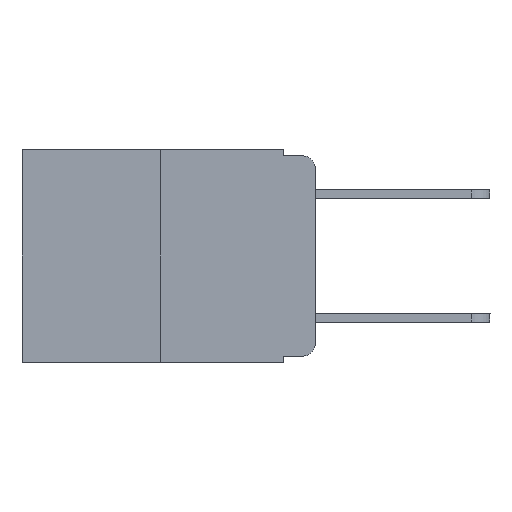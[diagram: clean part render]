
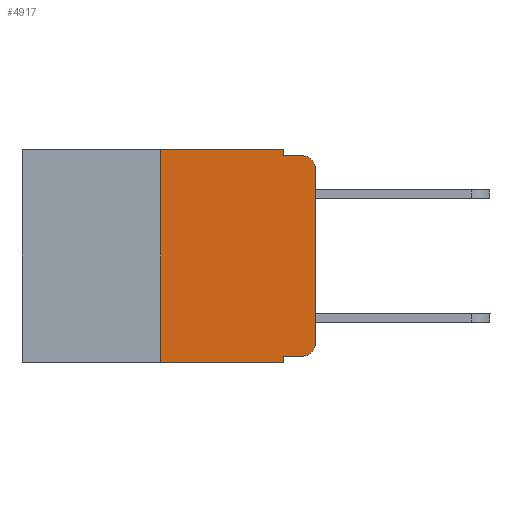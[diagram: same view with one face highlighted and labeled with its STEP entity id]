
A CAD part, left-side view. The second image highlights one B-rep face of the part: STEP entity #4917.
In plain terms, the highlighted planar face has unit normal (-1, 0, 0).
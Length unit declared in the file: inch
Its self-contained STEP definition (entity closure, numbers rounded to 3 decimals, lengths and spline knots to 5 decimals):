
#163 = ORIENTED_EDGE ( 'NONE', *, *, #10493, .F. ) ;
#191 = VERTEX_POINT ( 'NONE', #12729 ) ;
#669 = DIRECTION ( 'NONE',  ( 0., -1., 0. ) ) ;
#799 = VECTOR ( 'NONE', #8525, 39.37008 ) ;
#1104 = CARTESIAN_POINT ( 'NONE',  ( 0., 0.473, 0. ) ) ;
#1194 = ORIENTED_EDGE ( 'NONE', *, *, #16349, .T. ) ;
#1467 = VERTEX_POINT ( 'NONE', #7719 ) ;
#1587 = CARTESIAN_POINT ( 'NONE',  ( 0., 0., -0.03 ) ) ;
#1673 = LINE ( 'NONE', #8542, #1927 ) ;
#1927 = VECTOR ( 'NONE', #15159, 39.37008 ) ;
#2111 = EDGE_LOOP ( 'NONE', ( #20418, #5104, #2732, #8688, #163, #16193, #19515, #16951, #8560, #1194 ) ) ;
#2707 = EDGE_CURVE ( 'NONE', #16683, #191, #2872, .T. ) ;
#2732 = ORIENTED_EDGE ( 'NONE', *, *, #19059, .F. ) ;
#2756 = DIRECTION ( 'NONE',  ( 0., -1., 0. ) ) ;
#2762 = DIRECTION ( 'NONE',  ( 1., 0., 0. ) ) ;
#2872 = LINE ( 'NONE', #6411, #19790 ) ;
#3437 = CARTESIAN_POINT ( 'NONE',  ( 0., 0.051, -0.343 ) ) ;
#4051 = CARTESIAN_POINT ( 'NONE',  ( 0., 0., 0. ) ) ;
#4280 = VERTEX_POINT ( 'NONE', #19044 ) ;
#4456 = PLANE ( 'NONE',  #14859 ) ;
#4917 = ADVANCED_FACE ( 'NONE', ( #21011 ), #4456, .F. ) ;
#5104 = ORIENTED_EDGE ( 'NONE', *, *, #11301, .T. ) ;
#5699 = LINE ( 'NONE', #10876, #12565 ) ;
#5936 = VERTEX_POINT ( 'NONE', #19601 ) ;
#6309 = CARTESIAN_POINT ( 'NONE',  ( 0., 0.051, 0. ) ) ;
#6411 = CARTESIAN_POINT ( 'NONE',  ( 0., 0.25, 0. ) ) ;
#6610 = LINE ( 'NONE', #9608, #7412 ) ;
#6990 = LINE ( 'NONE', #10403, #10577 ) ;
#7412 = VECTOR ( 'NONE', #14306, 39.37008 ) ;
#7543 = LINE ( 'NONE', #12503, #9067 ) ;
#7676 = DIRECTION ( 'NONE',  ( 0., -1., 0. ) ) ;
#7719 = CARTESIAN_POINT ( 'NONE',  ( 0., 0.051, -0.01 ) ) ;
#8001 = CARTESIAN_POINT ( 'NONE',  ( 0., 0.25, -0.343 ) ) ;
#8077 = VERTEX_POINT ( 'NONE', #1587 ) ;
#8152 = DIRECTION ( 'NONE',  ( 0., 0., -1. ) ) ;
#8256 = EDGE_CURVE ( 'NONE', #4280, #21171, #1673, .T. ) ;
#8525 = DIRECTION ( 'NONE',  ( 0., -1., 0. ) ) ;
#8542 = CARTESIAN_POINT ( 'NONE',  ( 0., 0.051, 0. ) ) ;
#8560 = ORIENTED_EDGE ( 'NONE', *, *, #18444, .T. ) ;
#8688 = ORIENTED_EDGE ( 'NONE', *, *, #17361, .F. ) ;
#9067 = VECTOR ( 'NONE', #2756, 39.37008 ) ;
#9608 = CARTESIAN_POINT ( 'NONE',  ( 0., 0.051, 0. ) ) ;
#9983 = VERTEX_POINT ( 'NONE', #6309 ) ;
#10403 = CARTESIAN_POINT ( 'NONE',  ( 0., 0.473, -0.343 ) ) ;
#10416 = CARTESIAN_POINT ( 'NONE',  ( 0., 0.02, -0.01 ) ) ;
#10421 = CARTESIAN_POINT ( 'NONE',  ( 0., 0.473, 0. ) ) ;
#10491 = CARTESIAN_POINT ( 'NONE',  ( 0., 0., -0.313 ) ) ;
#10493 = EDGE_CURVE ( 'NONE', #191, #9983, #14091, .T. ) ;
#10577 = VECTOR ( 'NONE', #669, 39.37008 ) ;
#10876 = CARTESIAN_POINT ( 'NONE',  ( 0., 0.051, -0.01 ) ) ;
#11301 = EDGE_CURVE ( 'NONE', #8077, #13699, #20987, .T. ) ;
#12503 = CARTESIAN_POINT ( 'NONE',  ( 0., 0.051, -0.333 ) ) ;
#12565 = VECTOR ( 'NONE', #7676, 39.37008 ) ;
#12609 = EDGE_CURVE ( 'NONE', #13968, #8077, #20404, .T. ) ;
#12729 = CARTESIAN_POINT ( 'NONE',  ( 0., 0.25, 0. ) ) ;
#12872 = AXIS2_PLACEMENT_3D ( 'NONE', #17969, #16279, #8152 ) ;
#12905 = VECTOR ( 'NONE', #15463, 39.37008 ) ;
#13648 = AXIS2_PLACEMENT_3D ( 'NONE', #20213, #18488, #15290 ) ;
#13699 = VERTEX_POINT ( 'NONE', #10416 ) ;
#13968 = VERTEX_POINT ( 'NONE', #10491 ) ;
#14091 = LINE ( 'NONE', #10421, #799 ) ;
#14168 = DIRECTION ( 'NONE',  ( 0., 0., -1. ) ) ;
#14306 = DIRECTION ( 'NONE',  ( 0., 0., -1. ) ) ;
#14320 = EDGE_CURVE ( 'NONE', #16683, #21171, #6990, .T. ) ;
#14859 = AXIS2_PLACEMENT_3D ( 'NONE', #1104, #2762, #14168 ) ;
#15159 = DIRECTION ( 'NONE',  ( 0., 0., -1. ) ) ;
#15290 = DIRECTION ( 'NONE',  ( 0., 0., -1. ) ) ;
#15463 = DIRECTION ( 'NONE',  ( 0., 0., 1. ) ) ;
#16193 = ORIENTED_EDGE ( 'NONE', *, *, #2707, .F. ) ;
#16279 = DIRECTION ( 'NONE',  ( -1., 0., 0. ) ) ;
#16349 = EDGE_CURVE ( 'NONE', #5936, #13968, #20533, .T. ) ;
#16683 = VERTEX_POINT ( 'NONE', #8001 ) ;
#16951 = ORIENTED_EDGE ( 'NONE', *, *, #8256, .F. ) ;
#17361 = EDGE_CURVE ( 'NONE', #9983, #1467, #6610, .T. ) ;
#17808 = DIRECTION ( 'NONE',  ( 0., 0., 1. ) ) ;
#17969 = CARTESIAN_POINT ( 'NONE',  ( 0., 0.02, -0.03 ) ) ;
#18444 = EDGE_CURVE ( 'NONE', #4280, #5936, #7543, .T. ) ;
#18488 = DIRECTION ( 'NONE',  ( -1., 0., 0. ) ) ;
#19044 = CARTESIAN_POINT ( 'NONE',  ( 0., 0.051, -0.333 ) ) ;
#19059 = EDGE_CURVE ( 'NONE', #1467, #13699, #5699, .T. ) ;
#19515 = ORIENTED_EDGE ( 'NONE', *, *, #14320, .T. ) ;
#19601 = CARTESIAN_POINT ( 'NONE',  ( 0., 0.02, -0.333 ) ) ;
#19790 = VECTOR ( 'NONE', #17808, 39.37008 ) ;
#20213 = CARTESIAN_POINT ( 'NONE',  ( 0., 0.02, -0.313 ) ) ;
#20404 = LINE ( 'NONE', #4051, #12905 ) ;
#20418 = ORIENTED_EDGE ( 'NONE', *, *, #12609, .T. ) ;
#20533 = CIRCLE ( 'NONE', #13648, 0.02 ) ;
#20987 = CIRCLE ( 'NONE', #12872, 0.02 ) ;
#21011 = FACE_OUTER_BOUND ( 'NONE', #2111, .T. ) ;
#21171 = VERTEX_POINT ( 'NONE', #3437 ) ;
